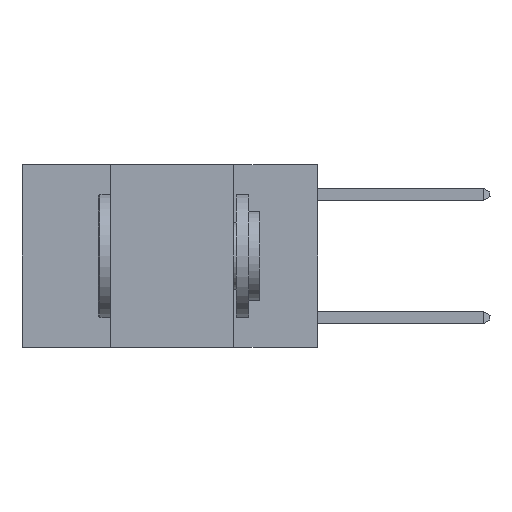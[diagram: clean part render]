
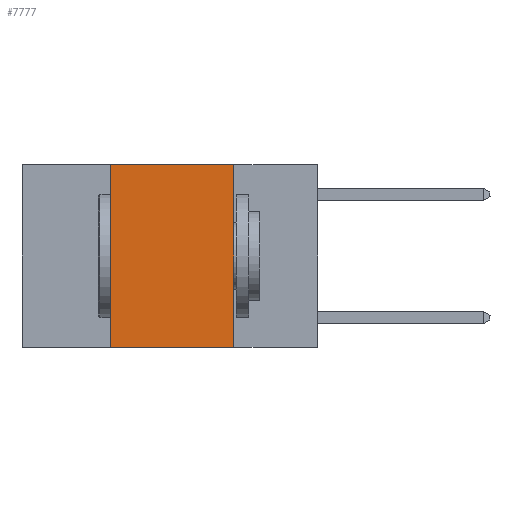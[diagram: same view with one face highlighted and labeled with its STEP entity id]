
A CAD part, left-side view. The second image highlights one B-rep face of the part: STEP entity #7777.
In plain terms, the highlighted planar face has unit normal (-1, 0, 0).
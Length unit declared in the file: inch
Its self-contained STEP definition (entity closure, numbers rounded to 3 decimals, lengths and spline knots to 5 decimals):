
#704 = DIRECTION ( 'NONE',  ( 0., -1., 0. ) ) ;
#1469 = CARTESIAN_POINT ( 'NONE',  ( 0., 0.17, 0. ) ) ;
#1624 = LINE ( 'NONE', #13957, #13892 ) ;
#1846 = VECTOR ( 'NONE', #9674, 39.37008 ) ;
#2191 = VECTOR ( 'NONE', #14704, 39.37008 ) ;
#2355 = CARTESIAN_POINT ( 'NONE',  ( 0., 0.6, 0. ) ) ;
#3733 = CARTESIAN_POINT ( 'NONE',  ( 0., 0.17, 0. ) ) ;
#4185 = ORIENTED_EDGE ( 'NONE', *, *, #9822, .T. ) ;
#4352 = LINE ( 'NONE', #2355, #1846 ) ;
#5412 = EDGE_CURVE ( 'NONE', #15734, #15433, #1624, .T. ) ;
#5451 = EDGE_LOOP ( 'NONE', ( #12757, #13152, #7033, #4185 ) ) ;
#6215 = DIRECTION ( 'NONE',  ( 0., 0., -1. ) ) ;
#7033 = ORIENTED_EDGE ( 'NONE', *, *, #5412, .F. ) ;
#7243 = AXIS2_PLACEMENT_3D ( 'NONE', #14694, #13552, #6215 ) ;
#7390 = CARTESIAN_POINT ( 'NONE',  ( 0., 0.42, -0.37 ) ) ;
#7777 = ADVANCED_FACE ( 'NONE', ( #15100 ), #13499, .F. ) ;
#7848 = DIRECTION ( 'NONE',  ( 0., 0., 1. ) ) ;
#8731 = CARTESIAN_POINT ( 'NONE',  ( 0., 0.17, -0.37 ) ) ;
#9674 = DIRECTION ( 'NONE',  ( 0., -1., 0. ) ) ;
#9822 = EDGE_CURVE ( 'NONE', #15734, #14133, #14122, .T. ) ;
#10771 = EDGE_CURVE ( 'NONE', #15433, #10974, #4352, .T. ) ;
#10872 = VECTOR ( 'NONE', #704, 39.37008 ) ;
#10974 = VERTEX_POINT ( 'NONE', #1469 ) ;
#11688 = CARTESIAN_POINT ( 'NONE',  ( 0., 0.6, -0.37 ) ) ;
#12108 = EDGE_CURVE ( 'NONE', #10974, #14133, #15148, .T. ) ;
#12757 = ORIENTED_EDGE ( 'NONE', *, *, #12108, .F. ) ;
#13152 = ORIENTED_EDGE ( 'NONE', *, *, #10771, .F. ) ;
#13499 = PLANE ( 'NONE',  #7243 ) ;
#13552 = DIRECTION ( 'NONE',  ( 1., 0., 0. ) ) ;
#13892 = VECTOR ( 'NONE', #7848, 39.37008 ) ;
#13957 = CARTESIAN_POINT ( 'NONE',  ( 0., 0.42, 0. ) ) ;
#14122 = LINE ( 'NONE', #11688, #10872 ) ;
#14133 = VERTEX_POINT ( 'NONE', #8731 ) ;
#14694 = CARTESIAN_POINT ( 'NONE',  ( 0., 0.6, 0. ) ) ;
#14704 = DIRECTION ( 'NONE',  ( 0., 0., -1. ) ) ;
#14727 = CARTESIAN_POINT ( 'NONE',  ( 0., 0.42, 0. ) ) ;
#15100 = FACE_OUTER_BOUND ( 'NONE', #5451, .T. ) ;
#15148 = LINE ( 'NONE', #3733, #2191 ) ;
#15433 = VERTEX_POINT ( 'NONE', #14727 ) ;
#15734 = VERTEX_POINT ( 'NONE', #7390 ) ;
